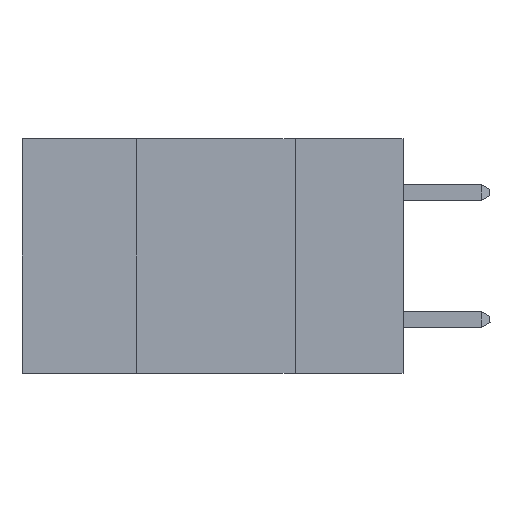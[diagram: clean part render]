
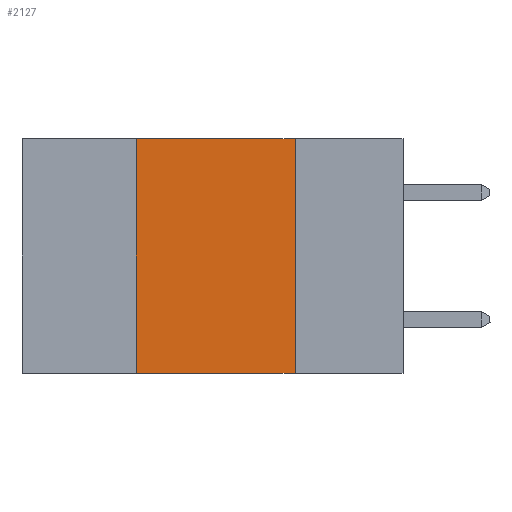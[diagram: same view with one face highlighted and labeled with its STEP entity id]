
A CAD part, left-side view. The second image highlights one B-rep face of the part: STEP entity #2127.
In plain terms, the highlighted planar face has unit normal (-1, 0, 0).
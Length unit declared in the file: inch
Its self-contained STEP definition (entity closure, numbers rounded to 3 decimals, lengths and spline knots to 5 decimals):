
#522 = CARTESIAN_POINT ( 'NONE',  ( 0., 0.42, -0.37 ) ) ;
#1009 = VERTEX_POINT ( 'NONE', #2179 ) ;
#1185 = CARTESIAN_POINT ( 'NONE',  ( 0., 0.17, 0. ) ) ;
#1623 = EDGE_CURVE ( 'NONE', #1626, #1009, #10560, .T. ) ;
#1626 = VERTEX_POINT ( 'NONE', #522 ) ;
#2127 = ADVANCED_FACE ( 'NONE', ( #5912 ), #14717, .F. ) ;
#2179 = CARTESIAN_POINT ( 'NONE',  ( 0., 0.42, 0. ) ) ;
#2213 = ORIENTED_EDGE ( 'NONE', *, *, #2248, .T. ) ;
#2248 = EDGE_CURVE ( 'NONE', #1626, #15044, #16477, .T. ) ;
#3340 = DIRECTION ( 'NONE',  ( 0., -1., 0. ) ) ;
#3357 = EDGE_CURVE ( 'NONE', #5707, #15044, #5221, .T. ) ;
#3711 = ORIENTED_EDGE ( 'NONE', *, *, #4053, .F. ) ;
#4053 = EDGE_CURVE ( 'NONE', #1009, #5707, #8165, .T. ) ;
#4101 = DIRECTION ( 'NONE',  ( 0., 0., -1. ) ) ;
#5221 = LINE ( 'NONE', #1185, #6489 ) ;
#5707 = VERTEX_POINT ( 'NONE', #6421 ) ;
#5912 = FACE_OUTER_BOUND ( 'NONE', #12535, .T. ) ;
#6086 = CARTESIAN_POINT ( 'NONE',  ( 0., 0.17, -0.37 ) ) ;
#6421 = CARTESIAN_POINT ( 'NONE',  ( 0., 0.17, 0. ) ) ;
#6489 = VECTOR ( 'NONE', #14639, 39.37008 ) ;
#8165 = LINE ( 'NONE', #12300, #9225 ) ;
#9225 = VECTOR ( 'NONE', #13648, 39.37008 ) ;
#9269 = VECTOR ( 'NONE', #3340, 39.37008 ) ;
#9763 = ORIENTED_EDGE ( 'NONE', *, *, #1623, .F. ) ;
#10560 = LINE ( 'NONE', #12699, #13328 ) ;
#11658 = CARTESIAN_POINT ( 'NONE',  ( 0., 0.6, -0.37 ) ) ;
#12300 = CARTESIAN_POINT ( 'NONE',  ( 0., 0.6, 0. ) ) ;
#12535 = EDGE_LOOP ( 'NONE', ( #16410, #3711, #9763, #2213 ) ) ;
#12699 = CARTESIAN_POINT ( 'NONE',  ( 0., 0.42, 0. ) ) ;
#13328 = VECTOR ( 'NONE', #16708, 39.37008 ) ;
#13648 = DIRECTION ( 'NONE',  ( 0., -1., 0. ) ) ;
#14639 = DIRECTION ( 'NONE',  ( 0., 0., -1. ) ) ;
#14717 = PLANE ( 'NONE',  #15134 ) ;
#15044 = VERTEX_POINT ( 'NONE', #6086 ) ;
#15134 = AXIS2_PLACEMENT_3D ( 'NONE', #17448, #15348, #4101 ) ;
#15348 = DIRECTION ( 'NONE',  ( 1., 0., 0. ) ) ;
#16410 = ORIENTED_EDGE ( 'NONE', *, *, #3357, .F. ) ;
#16477 = LINE ( 'NONE', #11658, #9269 ) ;
#16708 = DIRECTION ( 'NONE',  ( 0., 0., 1. ) ) ;
#17448 = CARTESIAN_POINT ( 'NONE',  ( 0., 0.6, 0. ) ) ;
